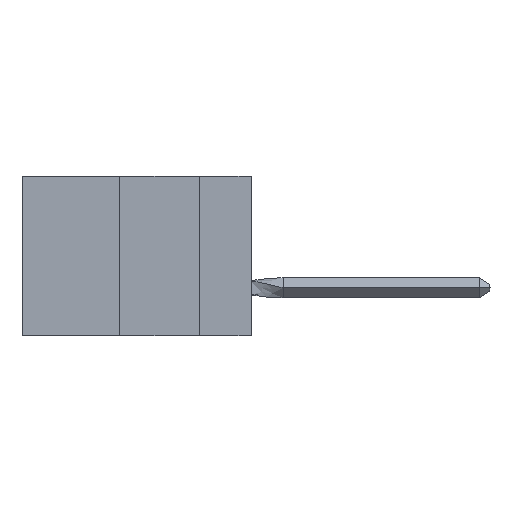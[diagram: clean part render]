
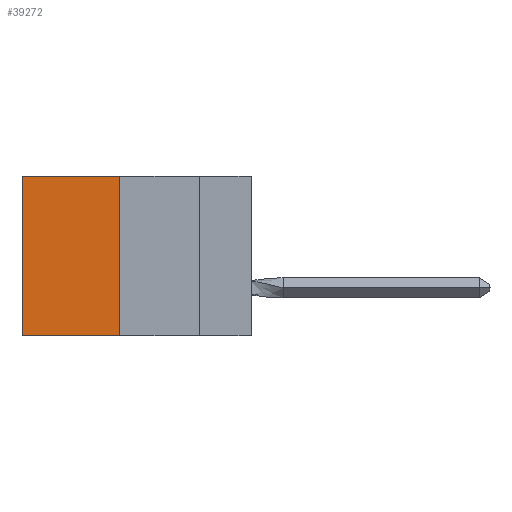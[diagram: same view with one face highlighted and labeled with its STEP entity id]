
A CAD part, left-side view. The second image highlights one B-rep face of the part: STEP entity #39272.
In plain terms, the highlighted planar face has unit normal (-1, 0, 0).
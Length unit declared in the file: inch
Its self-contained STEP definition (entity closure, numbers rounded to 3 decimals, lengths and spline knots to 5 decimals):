
#457 = VECTOR ( 'NONE', #30402, 39.37008 ) ;
#549 = CARTESIAN_POINT ( 'NONE',  ( 0.305, 0.72, 0. ) ) ;
#890 = VERTEX_POINT ( 'NONE', #28697 ) ;
#3186 = VECTOR ( 'NONE', #22586, 39.37008 ) ;
#3536 = EDGE_LOOP ( 'NONE', ( #17173, #37248, #31180, #6774 ) ) ;
#4443 = FACE_OUTER_BOUND ( 'NONE', #3536, .T. ) ;
#6458 = DIRECTION ( 'NONE',  ( 0., 0., -1. ) ) ;
#6774 = ORIENTED_EDGE ( 'NONE', *, *, #38691, .T. ) ;
#6851 = EDGE_CURVE ( 'NONE', #890, #22665, #37005, .T. ) ;
#7153 = VECTOR ( 'NONE', #12817, 39.37008 ) ;
#8146 = VERTEX_POINT ( 'NONE', #23868 ) ;
#9233 = CARTESIAN_POINT ( 'NONE',  ( 0.305, 0.72, -0.5 ) ) ;
#11252 = LINE ( 'NONE', #32241, #3186 ) ;
#11856 = LINE ( 'NONE', #27447, #18062 ) ;
#12817 = DIRECTION ( 'NONE',  ( 0., 1., 0. ) ) ;
#14079 = EDGE_CURVE ( 'NONE', #8146, #890, #11252, .T. ) ;
#15622 = PLANE ( 'NONE',  #35145 ) ;
#16604 = LINE ( 'NONE', #9233, #457 ) ;
#17173 = ORIENTED_EDGE ( 'NONE', *, *, #20522, .T. ) ;
#18062 = VECTOR ( 'NONE', #37259, 39.37008 ) ;
#20522 = EDGE_CURVE ( 'NONE', #27779, #22665, #16604, .T. ) ;
#22584 = CARTESIAN_POINT ( 'NONE',  ( 0.305, 0.72, -0.5 ) ) ;
#22586 = DIRECTION ( 'NONE',  ( 0., 0., -1. ) ) ;
#22665 = VERTEX_POINT ( 'NONE', #22584 ) ;
#23868 = CARTESIAN_POINT ( 'NONE',  ( 0.305, 0.413, 0. ) ) ;
#27447 = CARTESIAN_POINT ( 'NONE',  ( 0.305, 0.413, 0. ) ) ;
#27779 = VERTEX_POINT ( 'NONE', #549 ) ;
#28697 = CARTESIAN_POINT ( 'NONE',  ( 0.305, 0.413, -0.5 ) ) ;
#30402 = DIRECTION ( 'NONE',  ( 0., 0., -1. ) ) ;
#30549 = DIRECTION ( 'NONE',  ( 1., 0., 0. ) ) ;
#31180 = ORIENTED_EDGE ( 'NONE', *, *, #14079, .F. ) ;
#32241 = CARTESIAN_POINT ( 'NONE',  ( 0.305, 0.413, -0.5 ) ) ;
#33471 = CARTESIAN_POINT ( 'NONE',  ( 0.305, 0.413, -0.5 ) ) ;
#35145 = AXIS2_PLACEMENT_3D ( 'NONE', #36776, #30549, #6458 ) ;
#36776 = CARTESIAN_POINT ( 'NONE',  ( 0.305, 0.413, -0.5 ) ) ;
#37005 = LINE ( 'NONE', #33471, #7153 ) ;
#37248 = ORIENTED_EDGE ( 'NONE', *, *, #6851, .F. ) ;
#37259 = DIRECTION ( 'NONE',  ( 0., 1., 0. ) ) ;
#38691 = EDGE_CURVE ( 'NONE', #8146, #27779, #11856, .T. ) ;
#39272 = ADVANCED_FACE ( 'NONE', ( #4443 ), #15622, .F. ) ;
